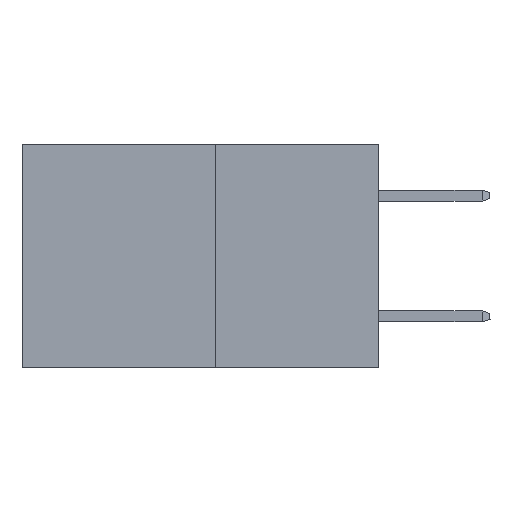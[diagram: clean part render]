
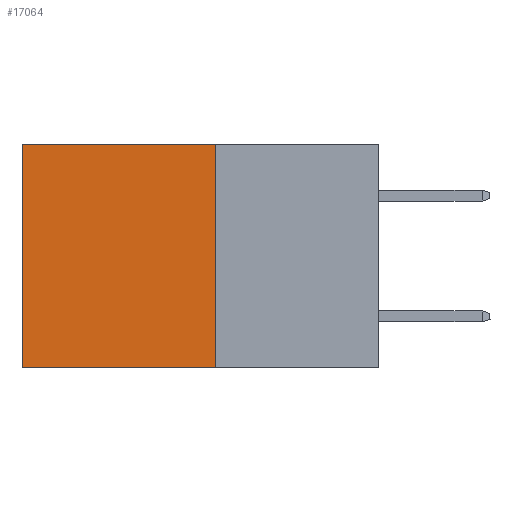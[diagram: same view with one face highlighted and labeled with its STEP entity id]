
A CAD part, left-side view. The second image highlights one B-rep face of the part: STEP entity #17064.
In plain terms, the highlighted planar face has unit normal (-1, 0, 0).
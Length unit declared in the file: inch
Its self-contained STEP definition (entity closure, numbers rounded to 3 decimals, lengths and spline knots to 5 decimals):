
#31 = DIRECTION ( 'NONE',  ( 0., 1., 0. ) ) ;
#132 = CARTESIAN_POINT ( 'NONE',  ( 0.277, 0.27, -0.37 ) ) ;
#314 = CARTESIAN_POINT ( 'NONE',  ( 0.277, 0.27, -0.37 ) ) ;
#1161 = CARTESIAN_POINT ( 'NONE',  ( 0.277, 0.59, 0. ) ) ;
#1174 = ORIENTED_EDGE ( 'NONE', *, *, #9084, .F. ) ;
#3274 = VERTEX_POINT ( 'NONE', #7851 ) ;
#3853 = VECTOR ( 'NONE', #17447, 39.37008 ) ;
#5223 = AXIS2_PLACEMENT_3D ( 'NONE', #19034, #8760, #20850 ) ;
#5566 = VERTEX_POINT ( 'NONE', #1161 ) ;
#5713 = VECTOR ( 'NONE', #31, 39.37008 ) ;
#5994 = FACE_OUTER_BOUND ( 'NONE', #15753, .T. ) ;
#6120 = ORIENTED_EDGE ( 'NONE', *, *, #17121, .F. ) ;
#7011 = PLANE ( 'NONE',  #5223 ) ;
#7851 = CARTESIAN_POINT ( 'NONE',  ( 0.277, 0.27, -0.37 ) ) ;
#8027 = EDGE_CURVE ( 'NONE', #5566, #17457, #22259, .T. ) ;
#8760 = DIRECTION ( 'NONE',  ( 1., 0., 0. ) ) ;
#8776 = ORIENTED_EDGE ( 'NONE', *, *, #8027, .T. ) ;
#9084 = EDGE_CURVE ( 'NONE', #3274, #17457, #18983, .T. ) ;
#9527 = VECTOR ( 'NONE', #10634, 39.37008 ) ;
#10131 = VERTEX_POINT ( 'NONE', #19519 ) ;
#10634 = DIRECTION ( 'NONE',  ( 0., 0., -1. ) ) ;
#11034 = LINE ( 'NONE', #11521, #19674 ) ;
#11521 = CARTESIAN_POINT ( 'NONE',  ( 0.277, 0.27, 0. ) ) ;
#11696 = DIRECTION ( 'NONE',  ( 0., 1., 0. ) ) ;
#14133 = LINE ( 'NONE', #314, #9527 ) ;
#14523 = EDGE_CURVE ( 'NONE', #10131, #5566, #11034, .T. ) ;
#15753 = EDGE_LOOP ( 'NONE', ( #8776, #1174, #6120, #18363 ) ) ;
#17064 = ADVANCED_FACE ( 'NONE', ( #5994 ), #7011, .F. ) ;
#17121 = EDGE_CURVE ( 'NONE', #10131, #3274, #14133, .T. ) ;
#17447 = DIRECTION ( 'NONE',  ( 0., 0., -1. ) ) ;
#17457 = VERTEX_POINT ( 'NONE', #21799 ) ;
#17616 = CARTESIAN_POINT ( 'NONE',  ( 0.277, 0.59, -0.37 ) ) ;
#18363 = ORIENTED_EDGE ( 'NONE', *, *, #14523, .T. ) ;
#18983 = LINE ( 'NONE', #132, #5713 ) ;
#19034 = CARTESIAN_POINT ( 'NONE',  ( 0.277, 0.27, -0.37 ) ) ;
#19519 = CARTESIAN_POINT ( 'NONE',  ( 0.277, 0.27, 0. ) ) ;
#19674 = VECTOR ( 'NONE', #11696, 39.37008 ) ;
#20850 = DIRECTION ( 'NONE',  ( 0., 0., -1. ) ) ;
#21799 = CARTESIAN_POINT ( 'NONE',  ( 0.277, 0.59, -0.37 ) ) ;
#22259 = LINE ( 'NONE', #17616, #3853 ) ;
